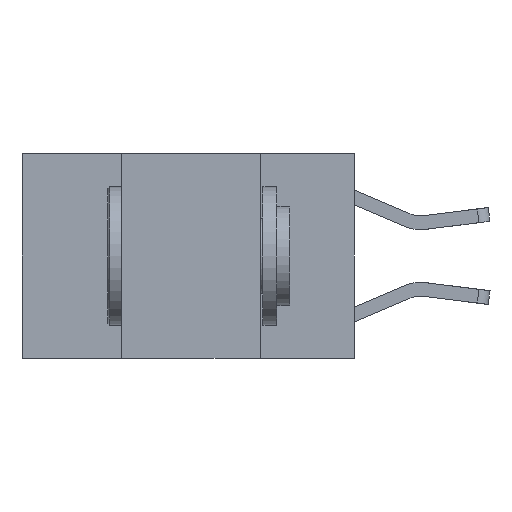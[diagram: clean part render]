
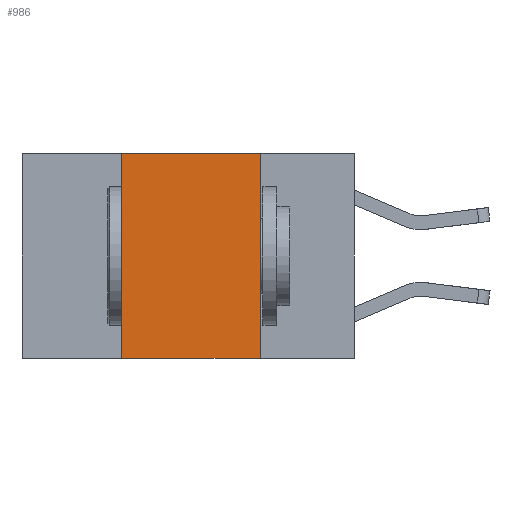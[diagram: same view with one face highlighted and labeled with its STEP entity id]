
A CAD part, left-side view. The second image highlights one B-rep face of the part: STEP entity #986.
In plain terms, the highlighted planar face has unit normal (-1, 0, 0).
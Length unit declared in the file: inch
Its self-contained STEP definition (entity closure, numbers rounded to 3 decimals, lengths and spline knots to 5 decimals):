
#228 = CARTESIAN_POINT ( 'NONE',  ( 0., 0.6, -0.37 ) ) ;
#401 = EDGE_LOOP ( 'NONE', ( #8701, #7875, #9198, #5752 ) ) ;
#481 = DIRECTION ( 'NONE',  ( 0., 0., 1. ) ) ;
#835 = VECTOR ( 'NONE', #481, 39.37008 ) ;
#887 = CARTESIAN_POINT ( 'NONE',  ( 0., 0.42, 0. ) ) ;
#986 = ADVANCED_FACE ( 'NONE', ( #8689 ), #3097, .F. ) ;
#2182 = CARTESIAN_POINT ( 'NONE',  ( 0., 0.17, 0. ) ) ;
#2372 = CARTESIAN_POINT ( 'NONE',  ( 0., 0.17, 0. ) ) ;
#2894 = DIRECTION ( 'NONE',  ( 0., 0., -1. ) ) ;
#3054 = DIRECTION ( 'NONE',  ( 1., 0., 0. ) ) ;
#3097 = PLANE ( 'NONE',  #5708 ) ;
#3779 = CARTESIAN_POINT ( 'NONE',  ( 0., 0.6, 0. ) ) ;
#4141 = LINE ( 'NONE', #2372, #10799 ) ;
#4261 = CARTESIAN_POINT ( 'NONE',  ( 0., 0.17, -0.37 ) ) ;
#4389 = CARTESIAN_POINT ( 'NONE',  ( 0., 0.42, -0.37 ) ) ;
#4895 = VECTOR ( 'NONE', #10144, 39.37008 ) ;
#5121 = CARTESIAN_POINT ( 'NONE',  ( 0., 0.42, 0. ) ) ;
#5547 = VERTEX_POINT ( 'NONE', #4261 ) ;
#5555 = EDGE_CURVE ( 'NONE', #9659, #10651, #5725, .T. ) ;
#5708 = AXIS2_PLACEMENT_3D ( 'NONE', #3779, #3054, #2894 ) ;
#5725 = LINE ( 'NONE', #5121, #835 ) ;
#5752 = ORIENTED_EDGE ( 'NONE', *, *, #6118, .T. ) ;
#5826 = VECTOR ( 'NONE', #9113, 39.37008 ) ;
#6118 = EDGE_CURVE ( 'NONE', #9659, #5547, #7495, .T. ) ;
#6510 = CARTESIAN_POINT ( 'NONE',  ( 0., 0.6, 0. ) ) ;
#6818 = EDGE_CURVE ( 'NONE', #10651, #10078, #10460, .T. ) ;
#7495 = LINE ( 'NONE', #228, #4895 ) ;
#7875 = ORIENTED_EDGE ( 'NONE', *, *, #6818, .F. ) ;
#8689 = FACE_OUTER_BOUND ( 'NONE', #401, .T. ) ;
#8701 = ORIENTED_EDGE ( 'NONE', *, *, #10200, .F. ) ;
#9113 = DIRECTION ( 'NONE',  ( 0., -1., 0. ) ) ;
#9198 = ORIENTED_EDGE ( 'NONE', *, *, #5555, .F. ) ;
#9659 = VERTEX_POINT ( 'NONE', #4389 ) ;
#10078 = VERTEX_POINT ( 'NONE', #2182 ) ;
#10144 = DIRECTION ( 'NONE',  ( 0., -1., 0. ) ) ;
#10200 = EDGE_CURVE ( 'NONE', #10078, #5547, #4141, .T. ) ;
#10460 = LINE ( 'NONE', #6510, #5826 ) ;
#10651 = VERTEX_POINT ( 'NONE', #887 ) ;
#10799 = VECTOR ( 'NONE', #11107, 39.37008 ) ;
#11107 = DIRECTION ( 'NONE',  ( 0., 0., -1. ) ) ;
